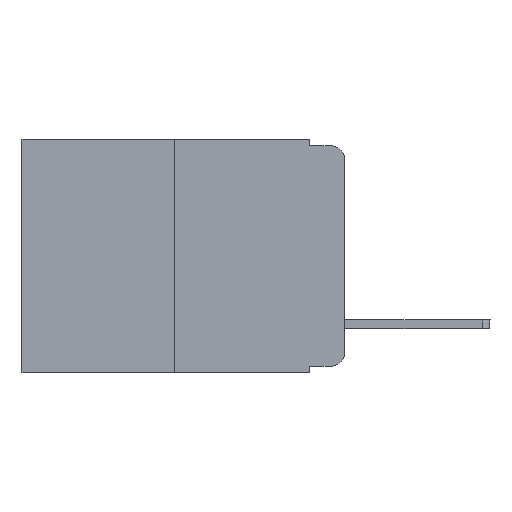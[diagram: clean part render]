
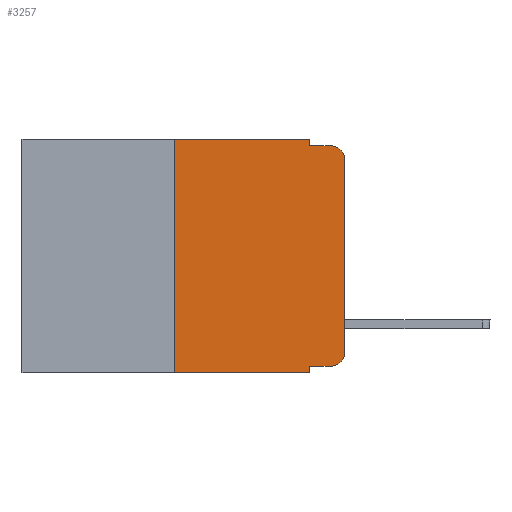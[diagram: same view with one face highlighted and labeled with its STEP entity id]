
A CAD part, left-side view. The second image highlights one B-rep face of the part: STEP entity #3257.
In plain terms, the highlighted planar face has unit normal (-1, 0, 0).
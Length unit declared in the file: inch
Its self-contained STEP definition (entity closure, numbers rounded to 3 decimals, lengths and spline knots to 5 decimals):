
#76 = ORIENTED_EDGE ( 'NONE', *, *, #480, .T. ) ;
#230 = VERTEX_POINT ( 'NONE', #8033 ) ;
#434 = VECTOR ( 'NONE', #6632, 39.37008 ) ;
#480 = EDGE_CURVE ( 'NONE', #6093, #230, #7004, .T. ) ;
#536 = DIRECTION ( 'NONE',  ( 0., -1., 0. ) ) ;
#590 = EDGE_CURVE ( 'NONE', #7883, #6947, #6806, .T. ) ;
#883 = CARTESIAN_POINT ( 'NONE',  ( 0., 0.473, 0. ) ) ;
#924 = CARTESIAN_POINT ( 'NONE',  ( 0., 0., -0.03 ) ) ;
#954 = DIRECTION ( 'NONE',  ( 0., -1., 0. ) ) ;
#980 = CARTESIAN_POINT ( 'NONE',  ( 0., 0.25, 0. ) ) ;
#985 = DIRECTION ( 'NONE',  ( -1., 0., 0. ) ) ;
#1024 = EDGE_CURVE ( 'NONE', #9301, #4992, #9992, .T. ) ;
#1074 = LINE ( 'NONE', #2540, #434 ) ;
#1160 = ORIENTED_EDGE ( 'NONE', *, *, #7566, .F. ) ;
#1188 = ORIENTED_EDGE ( 'NONE', *, *, #1024, .T. ) ;
#1189 = VERTEX_POINT ( 'NONE', #4941 ) ;
#1346 = VECTOR ( 'NONE', #6440, 39.37008 ) ;
#1445 = DIRECTION ( 'NONE',  ( 0., 0., -1. ) ) ;
#1963 = LINE ( 'NONE', #5142, #4565 ) ;
#2084 = ORIENTED_EDGE ( 'NONE', *, *, #590, .F. ) ;
#2109 = LINE ( 'NONE', #3684, #5230 ) ;
#2241 = VECTOR ( 'NONE', #954, 39.37008 ) ;
#2279 = ORIENTED_EDGE ( 'NONE', *, *, #4814, .F. ) ;
#2501 = FACE_OUTER_BOUND ( 'NONE', #3211, .T. ) ;
#2540 = CARTESIAN_POINT ( 'NONE',  ( 0., 0.473, -0.343 ) ) ;
#2874 = CARTESIAN_POINT ( 'NONE',  ( 0., 0.25, 0. ) ) ;
#2917 = CARTESIAN_POINT ( 'NONE',  ( 0., 0.051, 0. ) ) ;
#2996 = CARTESIAN_POINT ( 'NONE',  ( 0., 0.25, -0.343 ) ) ;
#3023 = ORIENTED_EDGE ( 'NONE', *, *, #3410, .T. ) ;
#3103 = DIRECTION ( 'NONE',  ( 0., -1., 0. ) ) ;
#3211 = EDGE_LOOP ( 'NONE', ( #3023, #1188, #6147, #4880, #1160, #2279, #5688, #2084, #5332, #76 ) ) ;
#3257 = ADVANCED_FACE ( 'NONE', ( #2501 ), #6646, .F. ) ;
#3410 = EDGE_CURVE ( 'NONE', #230, #9301, #1963, .T. ) ;
#3574 = DIRECTION ( 'NONE',  ( 0., 0., 1. ) ) ;
#3684 = CARTESIAN_POINT ( 'NONE',  ( 0., 0.051, 0. ) ) ;
#3756 = DIRECTION ( 'NONE',  ( -1., 0., 0. ) ) ;
#3832 = AXIS2_PLACEMENT_3D ( 'NONE', #5706, #985, #8894 ) ;
#4057 = CARTESIAN_POINT ( 'NONE',  ( 0., 0.051, -0.343 ) ) ;
#4565 = VECTOR ( 'NONE', #3574, 39.37008 ) ;
#4750 = CARTESIAN_POINT ( 'NONE',  ( 0., 0.02, -0.03 ) ) ;
#4814 = EDGE_CURVE ( 'NONE', #5968, #6012, #7998, .T. ) ;
#4852 = LINE ( 'NONE', #9434, #2241 ) ;
#4880 = ORIENTED_EDGE ( 'NONE', *, *, #7163, .F. ) ;
#4941 = CARTESIAN_POINT ( 'NONE',  ( 0., 0.051, 0. ) ) ;
#4992 = VERTEX_POINT ( 'NONE', #5114 ) ;
#5114 = CARTESIAN_POINT ( 'NONE',  ( 0., 0.02, -0.01 ) ) ;
#5142 = CARTESIAN_POINT ( 'NONE',  ( 0., 0., 0. ) ) ;
#5230 = VECTOR ( 'NONE', #6826, 39.37008 ) ;
#5332 = ORIENTED_EDGE ( 'NONE', *, *, #10180, .T. ) ;
#5411 = LINE ( 'NONE', #8594, #8955 ) ;
#5688 = ORIENTED_EDGE ( 'NONE', *, *, #9427, .T. ) ;
#5706 = CARTESIAN_POINT ( 'NONE',  ( 0., 0.02, -0.313 ) ) ;
#5751 = DIRECTION ( 'NONE',  ( 1., 0., 0. ) ) ;
#5848 = AXIS2_PLACEMENT_3D ( 'NONE', #4750, #3756, #1445 ) ;
#5968 = VERTEX_POINT ( 'NONE', #2996 ) ;
#6012 = VERTEX_POINT ( 'NONE', #2874 ) ;
#6017 = DIRECTION ( 'NONE',  ( 0., 0., -1. ) ) ;
#6093 = VERTEX_POINT ( 'NONE', #8646 ) ;
#6147 = ORIENTED_EDGE ( 'NONE', *, *, #8483, .F. ) ;
#6440 = DIRECTION ( 'NONE',  ( 0., 0., 1. ) ) ;
#6632 = DIRECTION ( 'NONE',  ( 0., -1., 0. ) ) ;
#6646 = PLANE ( 'NONE',  #8874 ) ;
#6806 = LINE ( 'NONE', #2917, #8672 ) ;
#6826 = DIRECTION ( 'NONE',  ( 0., 0., -1. ) ) ;
#6947 = VERTEX_POINT ( 'NONE', #4057 ) ;
#7004 = CIRCLE ( 'NONE', #3832, 0.02 ) ;
#7163 = EDGE_CURVE ( 'NONE', #1189, #8817, #2109, .T. ) ;
#7566 = EDGE_CURVE ( 'NONE', #6012, #1189, #10137, .T. ) ;
#7703 = CARTESIAN_POINT ( 'NONE',  ( 0., 0.473, 0. ) ) ;
#7883 = VERTEX_POINT ( 'NONE', #8456 ) ;
#7998 = LINE ( 'NONE', #980, #1346 ) ;
#8033 = CARTESIAN_POINT ( 'NONE',  ( 0., 0., -0.313 ) ) ;
#8239 = VECTOR ( 'NONE', #536, 39.37008 ) ;
#8456 = CARTESIAN_POINT ( 'NONE',  ( 0., 0.051, -0.333 ) ) ;
#8483 = EDGE_CURVE ( 'NONE', #8817, #4992, #4852, .T. ) ;
#8530 = CARTESIAN_POINT ( 'NONE',  ( 0., 0.051, -0.01 ) ) ;
#8594 = CARTESIAN_POINT ( 'NONE',  ( 0., 0.051, -0.333 ) ) ;
#8646 = CARTESIAN_POINT ( 'NONE',  ( 0., 0.02, -0.333 ) ) ;
#8672 = VECTOR ( 'NONE', #6017, 39.37008 ) ;
#8817 = VERTEX_POINT ( 'NONE', #8530 ) ;
#8874 = AXIS2_PLACEMENT_3D ( 'NONE', #883, #5751, #8945 ) ;
#8894 = DIRECTION ( 'NONE',  ( 0., 0., -1. ) ) ;
#8945 = DIRECTION ( 'NONE',  ( 0., 0., -1. ) ) ;
#8955 = VECTOR ( 'NONE', #3103, 39.37008 ) ;
#9301 = VERTEX_POINT ( 'NONE', #924 ) ;
#9427 = EDGE_CURVE ( 'NONE', #5968, #6947, #1074, .T. ) ;
#9434 = CARTESIAN_POINT ( 'NONE',  ( 0., 0.051, -0.01 ) ) ;
#9992 = CIRCLE ( 'NONE', #5848, 0.02 ) ;
#10137 = LINE ( 'NONE', #7703, #8239 ) ;
#10180 = EDGE_CURVE ( 'NONE', #7883, #6093, #5411, .T. ) ;
